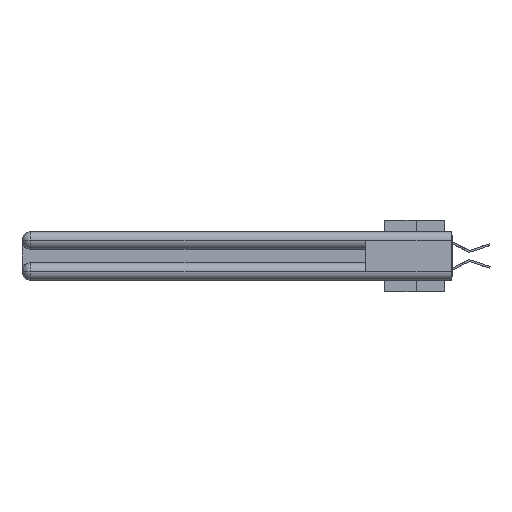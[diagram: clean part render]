
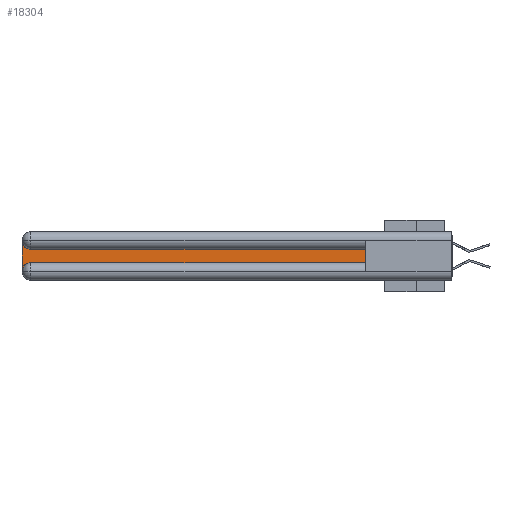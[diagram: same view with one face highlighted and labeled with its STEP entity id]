
A CAD part, left-side view. The second image highlights one B-rep face of the part: STEP entity #18304.
In plain terms, the highlighted planar face has unit normal (-1, 0, 0).
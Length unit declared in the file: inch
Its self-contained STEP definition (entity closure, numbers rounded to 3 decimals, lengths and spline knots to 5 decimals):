
#393 = CARTESIAN_POINT ( 'NONE',  ( 0.075, 2.94, -0.1225 ) ) ;
#513 = DIRECTION ( 'NONE',  ( 0., 0., -1. ) ) ;
#1705 = ORIENTED_EDGE ( 'NONE', *, *, #14834, .T. ) ;
#2895 = DIRECTION ( 'NONE',  ( 1., 0., 0. ) ) ;
#3799 = DIRECTION ( 'NONE',  ( 0., 1., 0. ) ) ;
#4529 = VECTOR ( 'NONE', #13584, 39.37008 ) ;
#4613 = EDGE_CURVE ( 'NONE', #24968, #19800, #36950, .T. ) ;
#5518 = DIRECTION ( 'NONE',  ( 1., 0., 0. ) ) ;
#5968 = DIRECTION ( 'NONE',  ( 0., -1., 0. ) ) ;
#6026 = CARTESIAN_POINT ( 'NONE',  ( 0.075, 2.94, -0.2775 ) ) ;
#7198 = ORIENTED_EDGE ( 'NONE', *, *, #37852, .T. ) ;
#7690 = AXIS2_PLACEMENT_3D ( 'NONE', #6026, #2895, #19427 ) ;
#8615 = VERTEX_POINT ( 'NONE', #24236 ) ;
#10228 = ORIENTED_EDGE ( 'NONE', *, *, #4613, .T. ) ;
#11213 = CARTESIAN_POINT ( 'NONE',  ( 0.075, 3., -0.2775 ) ) ;
#11946 = ORIENTED_EDGE ( 'NONE', *, *, #34660, .T. ) ;
#13315 = EDGE_CURVE ( 'NONE', #36385, #8615, #19744, .T. ) ;
#13584 = DIRECTION ( 'NONE',  ( 0., 0., 1. ) ) ;
#14834 = EDGE_CURVE ( 'NONE', #26325, #24968, #29905, .T. ) ;
#15348 = DIRECTION ( 'NONE',  ( 0., 0., -1. ) ) ;
#15631 = DIRECTION ( 'NONE',  ( 1., 0., 0. ) ) ;
#18304 = ADVANCED_FACE ( 'NONE', ( #28588 ), #22135, .F. ) ;
#18926 = AXIS2_PLACEMENT_3D ( 'NONE', #34387, #5518, #15348 ) ;
#19178 = ORIENTED_EDGE ( 'NONE', *, *, #13315, .T. ) ;
#19427 = DIRECTION ( 'NONE',  ( 0., 0., -1. ) ) ;
#19477 = CARTESIAN_POINT ( 'NONE',  ( 0.075, 0.6, -0.1225 ) ) ;
#19744 = CIRCLE ( 'NONE', #7690, 0.06 ) ;
#19800 = VERTEX_POINT ( 'NONE', #39538 ) ;
#22135 = PLANE ( 'NONE',  #27282 ) ;
#22334 = EDGE_CURVE ( 'NONE', #29966, #26325, #35951, .T. ) ;
#24236 = CARTESIAN_POINT ( 'NONE',  ( 0.075, 2.94, -0.2175 ) ) ;
#24968 = VERTEX_POINT ( 'NONE', #393 ) ;
#26325 = VERTEX_POINT ( 'NONE', #19477 ) ;
#27282 = AXIS2_PLACEMENT_3D ( 'NONE', #31710, #15631, #37815 ) ;
#27712 = LINE ( 'NONE', #34636, #30994 ) ;
#27855 = ORIENTED_EDGE ( 'NONE', *, *, #22334, .T. ) ;
#28588 = FACE_OUTER_BOUND ( 'NONE', #30531, .T. ) ;
#29157 = CARTESIAN_POINT ( 'NONE',  ( 0.075, 3., -0.2175 ) ) ;
#29905 = LINE ( 'NONE', #39336, #31841 ) ;
#29966 = VERTEX_POINT ( 'NONE', #35763 ) ;
#30531 = EDGE_LOOP ( 'NONE', ( #1705, #10228, #7198, #19178, #11946, #27855 ) ) ;
#30994 = VECTOR ( 'NONE', #5968, 39.37008 ) ;
#31710 = CARTESIAN_POINT ( 'NONE',  ( 0.075, 3., -0.1225 ) ) ;
#31841 = VECTOR ( 'NONE', #3799, 39.37008 ) ;
#34387 = CARTESIAN_POINT ( 'NONE',  ( 0.075, 2.94, -0.0625 ) ) ;
#34636 = CARTESIAN_POINT ( 'NONE',  ( 0.075, 0.6, -0.2175 ) ) ;
#34660 = EDGE_CURVE ( 'NONE', #8615, #29966, #27712, .T. ) ;
#35338 = CARTESIAN_POINT ( 'NONE',  ( 0.075, 0.6, -0.2175 ) ) ;
#35763 = CARTESIAN_POINT ( 'NONE',  ( 0.075, 0.6, -0.2175 ) ) ;
#35951 = LINE ( 'NONE', #35338, #4529 ) ;
#36385 = VERTEX_POINT ( 'NONE', #11213 ) ;
#36950 = CIRCLE ( 'NONE', #18926, 0.06 ) ;
#37815 = DIRECTION ( 'NONE',  ( 0., 0., -1. ) ) ;
#37852 = EDGE_CURVE ( 'NONE', #19800, #36385, #39205, .T. ) ;
#39205 = LINE ( 'NONE', #29157, #39476 ) ;
#39336 = CARTESIAN_POINT ( 'NONE',  ( 0.075, 0.6, -0.1225 ) ) ;
#39476 = VECTOR ( 'NONE', #513, 39.37008 ) ;
#39538 = CARTESIAN_POINT ( 'NONE',  ( 0.075, 3., -0.0625 ) ) ;
